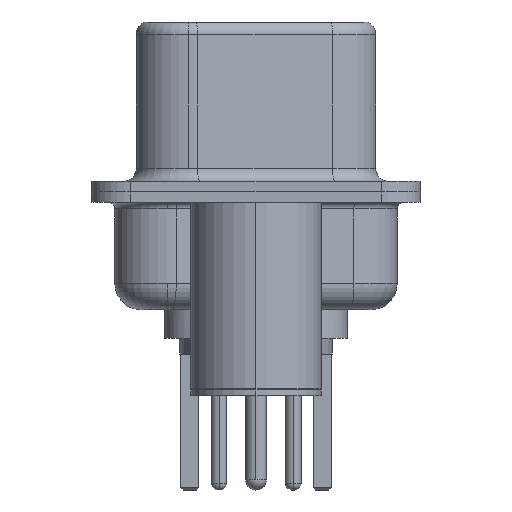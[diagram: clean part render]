
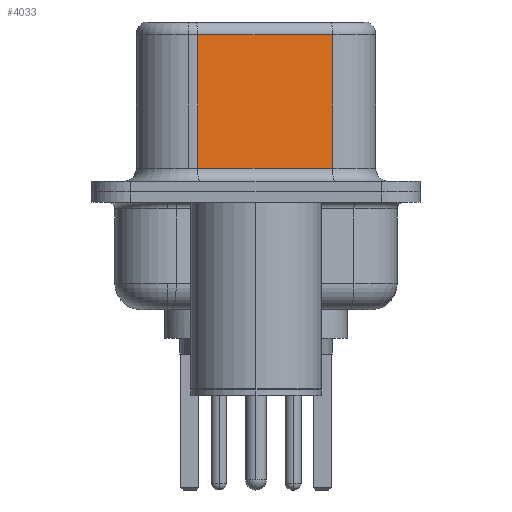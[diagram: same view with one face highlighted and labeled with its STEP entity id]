
A CAD part, left-side view. The second image highlights one B-rep face of the part: STEP entity #4033.
In plain terms, the highlighted planar face has unit normal (-0.985, -0.174, 0).
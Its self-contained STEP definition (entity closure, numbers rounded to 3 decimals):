
#1368 = VERTEX_POINT ( 'NONE', #20764 ) ;
#1397 = DIRECTION ( 'NONE',  ( 0., 0., -1. ) ) ;
#1604 = PLANE ( 'NONE',  #22121 ) ;
#1620 = DIRECTION ( 'NONE',  ( 0.174, -0.985, 0. ) ) ;
#2021 = LINE ( 'NONE', #22033, #10251 ) ;
#2672 = CARTESIAN_POINT ( 'NONE',  ( 3.655, 2.233, 0.9 ) ) ;
#2897 = ORIENTED_EDGE ( 'NONE', *, *, #4934, .T. ) ;
#4033 = ADVANCED_FACE ( 'NONE', ( #10672 ), #1604, .F. ) ;
#4678 = LINE ( 'NONE', #16216, #8496 ) ;
#4934 = EDGE_CURVE ( 'NONE', #5286, #1368, #20308, .T. ) ;
#5286 = VERTEX_POINT ( 'NONE', #15607 ) ;
#6003 = EDGE_CURVE ( 'NONE', #5286, #18714, #4678, .T. ) ;
#6182 = CARTESIAN_POINT ( 'NONE',  ( 3.655, 2.233, 6.52 ) ) ;
#6349 = DIRECTION ( 'NONE',  ( 0.985, 0.174, 0. ) ) ;
#7122 = EDGE_CURVE ( 'NONE', #11656, #18714, #2021, .T. ) ;
#7991 = CARTESIAN_POINT ( 'NONE',  ( 4.565, -2.927, 0.9 ) ) ;
#8496 = VECTOR ( 'NONE', #1397, 1000. ) ;
#8500 = DIRECTION ( 'NONE',  ( -0.174, 0.985, 0. ) ) ;
#8521 = CARTESIAN_POINT ( 'NONE',  ( 4.565, -2.927, 6.02 ) ) ;
#9546 = EDGE_CURVE ( 'NONE', #1368, #11656, #17027, .T. ) ;
#9912 = EDGE_LOOP ( 'NONE', ( #21227, #2897, #12624, #20706 ) ) ;
#10251 = VECTOR ( 'NONE', #1620, 1000. ) ;
#10672 = FACE_OUTER_BOUND ( 'NONE', #9912, .T. ) ;
#11656 = VERTEX_POINT ( 'NONE', #2672 ) ;
#12206 = VECTOR ( 'NONE', #20832, 1000. ) ;
#12624 = ORIENTED_EDGE ( 'NONE', *, *, #9546, .T. ) ;
#15233 = DIRECTION ( 'NONE',  ( -0.174, 0.985, 0. ) ) ;
#15445 = VECTOR ( 'NONE', #8500, 1000. ) ;
#15607 = CARTESIAN_POINT ( 'NONE',  ( 4.565, -2.927, 6.02 ) ) ;
#16216 = CARTESIAN_POINT ( 'NONE',  ( 4.565, -2.927, 6.52 ) ) ;
#17027 = LINE ( 'NONE', #6182, #12206 ) ;
#18714 = VERTEX_POINT ( 'NONE', #7991 ) ;
#20308 = LINE ( 'NONE', #8521, #15445 ) ;
#20456 = CARTESIAN_POINT ( 'NONE',  ( 4.565, -2.927, 6.52 ) ) ;
#20706 = ORIENTED_EDGE ( 'NONE', *, *, #7122, .T. ) ;
#20764 = CARTESIAN_POINT ( 'NONE',  ( 3.655, 2.233, 6.02 ) ) ;
#20832 = DIRECTION ( 'NONE',  ( 0., 0., -1. ) ) ;
#21227 = ORIENTED_EDGE ( 'NONE', *, *, #6003, .F. ) ;
#22033 = CARTESIAN_POINT ( 'NONE',  ( 4.565, -2.927, 0.9 ) ) ;
#22121 = AXIS2_PLACEMENT_3D ( 'NONE', #20456, #6349, #15233 ) ;
